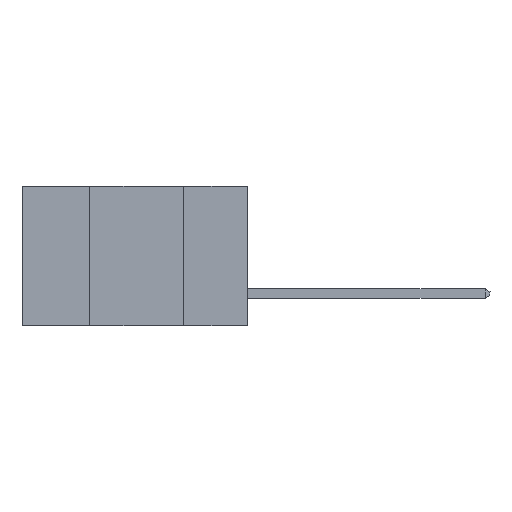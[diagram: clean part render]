
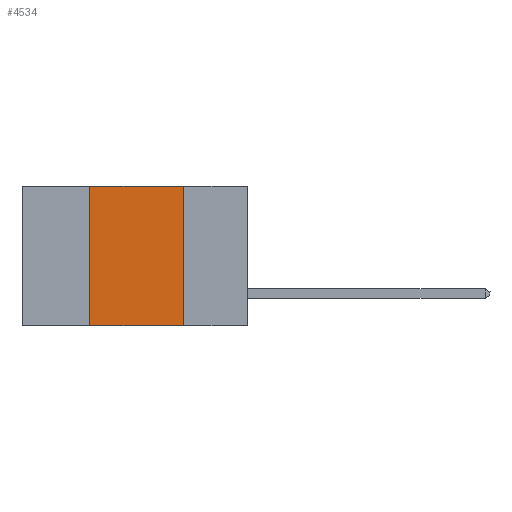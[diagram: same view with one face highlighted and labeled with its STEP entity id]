
A CAD part, left-side view. The second image highlights one B-rep face of the part: STEP entity #4534.
In plain terms, the highlighted planar face has unit normal (-1, 0, 0).
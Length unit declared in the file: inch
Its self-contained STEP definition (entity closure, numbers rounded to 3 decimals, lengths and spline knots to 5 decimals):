
#13 = VECTOR ( 'NONE', #1879, 39.37008 ) ;
#187 = CARTESIAN_POINT ( 'NONE',  ( 0., 0.17, -0.37 ) ) ;
#851 = CARTESIAN_POINT ( 'NONE',  ( 0., 0.17, -0.37 ) ) ;
#1013 = CARTESIAN_POINT ( 'NONE',  ( 0., 0.42, 0. ) ) ;
#1533 = AXIS2_PLACEMENT_3D ( 'NONE', #7120, #3168, #9665 ) ;
#1709 = CARTESIAN_POINT ( 'NONE',  ( 0., 0.42, -0.37 ) ) ;
#1820 = LINE ( 'NONE', #1709, #5387 ) ;
#1879 = DIRECTION ( 'NONE',  ( 0., 0., -1. ) ) ;
#1968 = LINE ( 'NONE', #3573, #7828 ) ;
#2007 = CARTESIAN_POINT ( 'NONE',  ( 0., 0.6, 0. ) ) ;
#3092 = VERTEX_POINT ( 'NONE', #9780 ) ;
#3168 = DIRECTION ( 'NONE',  ( 1., 0., 0. ) ) ;
#3280 = ORIENTED_EDGE ( 'NONE', *, *, #4610, .F. ) ;
#3526 = EDGE_CURVE ( 'NONE', #4086, #5653, #1820, .T. ) ;
#3573 = CARTESIAN_POINT ( 'NONE',  ( 0., 0.6, -0.37 ) ) ;
#4086 = VERTEX_POINT ( 'NONE', #7730 ) ;
#4411 = LINE ( 'NONE', #2007, #9152 ) ;
#4534 = ADVANCED_FACE ( 'NONE', ( #9460 ), #7218, .F. ) ;
#4610 = EDGE_CURVE ( 'NONE', #3092, #4777, #6537, .T. ) ;
#4777 = VERTEX_POINT ( 'NONE', #851 ) ;
#5120 = ORIENTED_EDGE ( 'NONE', *, *, #3526, .F. ) ;
#5387 = VECTOR ( 'NONE', #8083, 39.37008 ) ;
#5653 = VERTEX_POINT ( 'NONE', #1013 ) ;
#6157 = DIRECTION ( 'NONE',  ( 0., -1., 0. ) ) ;
#6416 = ORIENTED_EDGE ( 'NONE', *, *, #10312, .T. ) ;
#6537 = LINE ( 'NONE', #187, #13 ) ;
#7014 = EDGE_CURVE ( 'NONE', #5653, #3092, #4411, .T. ) ;
#7120 = CARTESIAN_POINT ( 'NONE',  ( 0., 0.6, 0. ) ) ;
#7218 = PLANE ( 'NONE',  #1533 ) ;
#7730 = CARTESIAN_POINT ( 'NONE',  ( 0., 0.42, -0.37 ) ) ;
#7828 = VECTOR ( 'NONE', #9930, 39.37008 ) ;
#8083 = DIRECTION ( 'NONE',  ( 0., 0., 1. ) ) ;
#9118 = ORIENTED_EDGE ( 'NONE', *, *, #7014, .F. ) ;
#9152 = VECTOR ( 'NONE', #6157, 39.37008 ) ;
#9165 = EDGE_LOOP ( 'NONE', ( #3280, #9118, #5120, #6416 ) ) ;
#9460 = FACE_OUTER_BOUND ( 'NONE', #9165, .T. ) ;
#9665 = DIRECTION ( 'NONE',  ( 0., 0., -1. ) ) ;
#9780 = CARTESIAN_POINT ( 'NONE',  ( 0., 0.17, 0. ) ) ;
#9930 = DIRECTION ( 'NONE',  ( 0., -1., 0. ) ) ;
#10312 = EDGE_CURVE ( 'NONE', #4086, #4777, #1968, .T. ) ;
